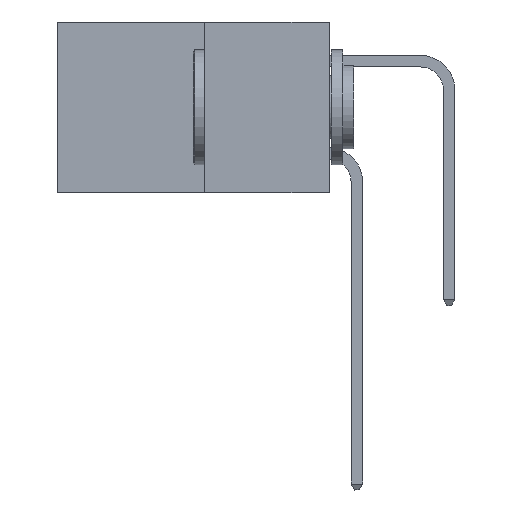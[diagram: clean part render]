
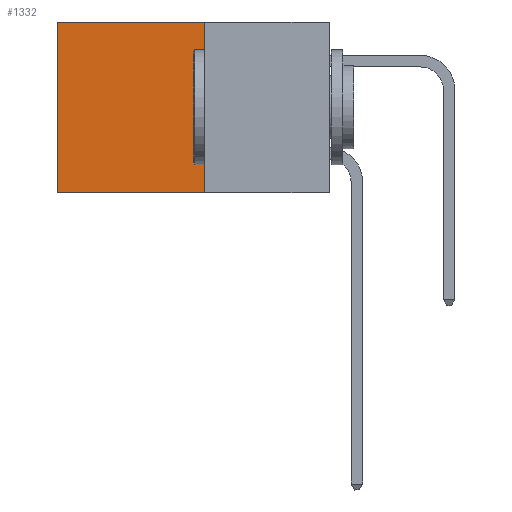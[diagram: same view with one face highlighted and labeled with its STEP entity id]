
A CAD part, left-side view. The second image highlights one B-rep face of the part: STEP entity #1332.
In plain terms, the highlighted planar face has unit normal (-1, 0, 0).
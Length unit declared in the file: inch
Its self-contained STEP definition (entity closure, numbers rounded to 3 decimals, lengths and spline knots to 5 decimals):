
#42 = ORIENTED_EDGE ( 'NONE', *, *, #9355, .T. ) ;
#153 = LINE ( 'NONE', #3987, #8816 ) ;
#445 = VECTOR ( 'NONE', #2826, 39.37008 ) ;
#1119 = AXIS2_PLACEMENT_3D ( 'NONE', #9031, #2415, #2977 ) ;
#1332 = ADVANCED_FACE ( 'NONE', ( #8905 ), #7966, .F. ) ;
#1349 = ORIENTED_EDGE ( 'NONE', *, *, #10453, .F. ) ;
#1954 = CARTESIAN_POINT ( 'NONE',  ( 0.277, 0.27, 0. ) ) ;
#2415 = DIRECTION ( 'NONE',  ( 1., 0., 0. ) ) ;
#2504 = VECTOR ( 'NONE', #5684, 39.37008 ) ;
#2826 = DIRECTION ( 'NONE',  ( 0., 1., 0. ) ) ;
#2890 = LINE ( 'NONE', #1954, #445 ) ;
#2977 = DIRECTION ( 'NONE',  ( 0., 0., -1. ) ) ;
#3095 = CARTESIAN_POINT ( 'NONE',  ( 0.277, 0.59, 0. ) ) ;
#3413 = VERTEX_POINT ( 'NONE', #9024 ) ;
#3515 = ORIENTED_EDGE ( 'NONE', *, *, #8464, .F. ) ;
#3987 = CARTESIAN_POINT ( 'NONE',  ( 0.277, 0.27, -0.37 ) ) ;
#4072 = CARTESIAN_POINT ( 'NONE',  ( 0.277, 0.59, -0.37 ) ) ;
#4138 = EDGE_LOOP ( 'NONE', ( #7344, #3515, #1349, #42 ) ) ;
#4922 = EDGE_CURVE ( 'NONE', #8840, #4940, #6828, .T. ) ;
#4940 = VERTEX_POINT ( 'NONE', #4072 ) ;
#5183 = CARTESIAN_POINT ( 'NONE',  ( 0.277, 0.27, -0.37 ) ) ;
#5684 = DIRECTION ( 'NONE',  ( 0., 0., -1. ) ) ;
#6828 = LINE ( 'NONE', #8114, #2504 ) ;
#7344 = ORIENTED_EDGE ( 'NONE', *, *, #4922, .T. ) ;
#7854 = VECTOR ( 'NONE', #8435, 39.37008 ) ;
#7966 = PLANE ( 'NONE',  #1119 ) ;
#8114 = CARTESIAN_POINT ( 'NONE',  ( 0.277, 0.59, -0.37 ) ) ;
#8435 = DIRECTION ( 'NONE',  ( 0., 1., 0. ) ) ;
#8464 = EDGE_CURVE ( 'NONE', #10460, #4940, #9923, .T. ) ;
#8816 = VECTOR ( 'NONE', #9588, 39.37008 ) ;
#8840 = VERTEX_POINT ( 'NONE', #3095 ) ;
#8905 = FACE_OUTER_BOUND ( 'NONE', #4138, .T. ) ;
#9024 = CARTESIAN_POINT ( 'NONE',  ( 0.277, 0.27, 0. ) ) ;
#9031 = CARTESIAN_POINT ( 'NONE',  ( 0.277, 0.27, -0.37 ) ) ;
#9355 = EDGE_CURVE ( 'NONE', #3413, #8840, #2890, .T. ) ;
#9588 = DIRECTION ( 'NONE',  ( 0., 0., -1. ) ) ;
#9923 = LINE ( 'NONE', #5183, #7854 ) ;
#10355 = CARTESIAN_POINT ( 'NONE',  ( 0.277, 0.27, -0.37 ) ) ;
#10453 = EDGE_CURVE ( 'NONE', #3413, #10460, #153, .T. ) ;
#10460 = VERTEX_POINT ( 'NONE', #10355 ) ;
